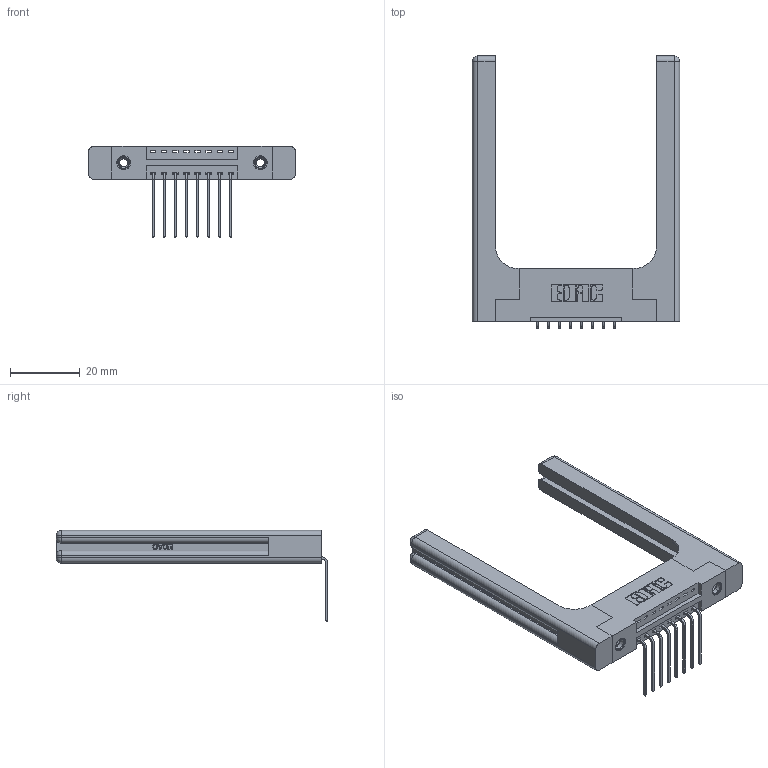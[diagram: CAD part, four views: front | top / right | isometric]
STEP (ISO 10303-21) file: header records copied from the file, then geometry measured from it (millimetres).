
FILE_DESCRIPTION (( 'STEP AP203' ), '1' );
FILE_NAME ('346-008-559-158.STEP', '2022-05-04T21:41:58', ( '' ), ( '' ), 'SwSTEP 2.0', 'SolidWorks 2020', '' );
FILE_SCHEMA (( 'CONFIG_CONTROL_DESIGN' ));
Length unit declared in the file: inch
Products named in the file (5): 345-292-001_558 559 Tail - 1; 345-250-001_345-250-001-102; 346-008-559-158; 346 Part_Flush Mounting Lugs - 0.156 Dia-TH; 346-220-058_345-220-058
Assembly tree (13 placements, depth 2):
  346-008-559-158
    346 Part_Flush Mounting Lugs - 0.156 Dia-TH
    345-292-001_558 559 Tail - 1  x8
    345-250-001_345-250-001-102  x2
    346-220-058_345-220-058  x2
Bounding box: 59.46 x 78.04 x 26.16 mm (x, y, z)
Volume: 12984.5 mm3; surface area: 11825.8 mm2
Topology: 13 solids, 13 shells, 872 faces, 2487 edges, 1626 vertices
Faces by surface type: plane 574, cylinder 238, bspline 36, cone 12, sphere 8, torus 4
Entity records: 15224 total; most frequent: CARTESIAN_POINT 3603, ORIENTED_EDGE 2340, DIRECTION 2150, EDGE_CURVE 1170, LINE 914, VECTOR 914, VERTEX_POINT 770, AXIS2_PLACEMENT_3D 618
